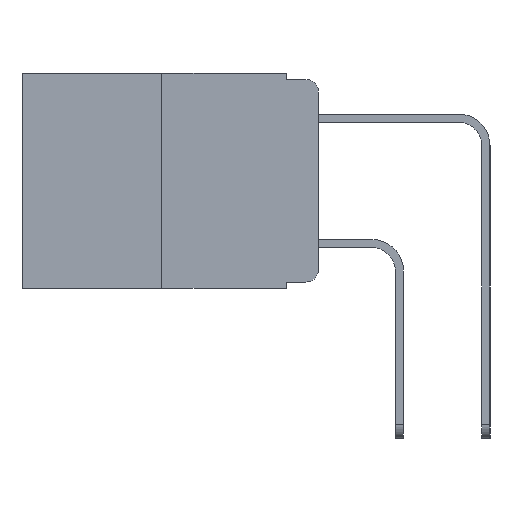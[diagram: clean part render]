
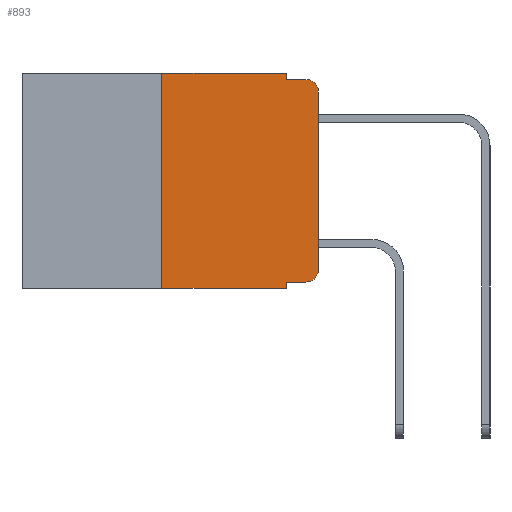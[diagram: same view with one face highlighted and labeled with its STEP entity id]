
A CAD part, left-side view. The second image highlights one B-rep face of the part: STEP entity #893.
In plain terms, the highlighted planar face has unit normal (-1, 0, 0).
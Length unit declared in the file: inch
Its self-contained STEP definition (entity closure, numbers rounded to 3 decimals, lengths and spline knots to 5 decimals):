
#57 = ORIENTED_EDGE ( 'NONE', *, *, #6435, .F. ) ;
#173 = CARTESIAN_POINT ( 'NONE',  ( 0., 0.051, -0.01 ) ) ;
#435 = DIRECTION ( 'NONE',  ( 0., 0., 1. ) ) ;
#617 = DIRECTION ( 'NONE',  ( 0., 0., -1. ) ) ;
#740 = DIRECTION ( 'NONE',  ( 0., -1., 0. ) ) ;
#786 = ORIENTED_EDGE ( 'NONE', *, *, #6871, .T. ) ;
#841 = ORIENTED_EDGE ( 'NONE', *, *, #5917, .T. ) ;
#893 = ADVANCED_FACE ( 'NONE', ( #14745 ), #947, .F. ) ;
#947 = PLANE ( 'NONE',  #5360 ) ;
#1218 = EDGE_CURVE ( 'NONE', #14982, #10370, #7694, .T. ) ;
#1317 = VECTOR ( 'NONE', #435, 39.37008 ) ;
#1763 = EDGE_LOOP ( 'NONE', ( #786, #841, #57, #3792, #8939, #8729, #2257, #1933, #3861, #8862 ) ) ;
#1921 = CIRCLE ( 'NONE', #11222, 0.02 ) ;
#1933 = ORIENTED_EDGE ( 'NONE', *, *, #4482, .F. ) ;
#2257 = ORIENTED_EDGE ( 'NONE', *, *, #1218, .T. ) ;
#2333 = DIRECTION ( 'NONE',  ( 0., 0., -1. ) ) ;
#2647 = CARTESIAN_POINT ( 'NONE',  ( 0., 0.02, -0.03 ) ) ;
#3167 = CARTESIAN_POINT ( 'NONE',  ( 0., 0., 0. ) ) ;
#3322 = CARTESIAN_POINT ( 'NONE',  ( 0., 0.02, -0.01 ) ) ;
#3792 = ORIENTED_EDGE ( 'NONE', *, *, #13071, .F. ) ;
#3861 = ORIENTED_EDGE ( 'NONE', *, *, #12521, .T. ) ;
#3961 = DIRECTION ( 'NONE',  ( 0., 0., -1. ) ) ;
#4212 = LINE ( 'NONE', #9651, #7552 ) ;
#4482 = EDGE_CURVE ( 'NONE', #14192, #10370, #9953, .T. ) ;
#4550 = CARTESIAN_POINT ( 'NONE',  ( 0., 0.02, -0.333 ) ) ;
#4889 = CIRCLE ( 'NONE', #15870, 0.02 ) ;
#4907 = DIRECTION ( 'NONE',  ( 1., 0., 0. ) ) ;
#4978 = VERTEX_POINT ( 'NONE', #3322 ) ;
#5306 = VERTEX_POINT ( 'NONE', #9014 ) ;
#5360 = AXIS2_PLACEMENT_3D ( 'NONE', #11099, #4907, #13503 ) ;
#5851 = DIRECTION ( 'NONE',  ( 0., -1., 0. ) ) ;
#5917 = EDGE_CURVE ( 'NONE', #10586, #4978, #1921, .T. ) ;
#6300 = CARTESIAN_POINT ( 'NONE',  ( 0., 0.051, 0. ) ) ;
#6374 = DIRECTION ( 'NONE',  ( -1., 0., 0. ) ) ;
#6435 = EDGE_CURVE ( 'NONE', #14594, #4978, #11565, .T. ) ;
#6600 = VECTOR ( 'NONE', #2333, 39.37008 ) ;
#6871 = EDGE_CURVE ( 'NONE', #10954, #10586, #8699, .T. ) ;
#7233 = LINE ( 'NONE', #9596, #10561 ) ;
#7552 = VECTOR ( 'NONE', #10809, 39.37008 ) ;
#7694 = LINE ( 'NONE', #8012, #13799 ) ;
#8012 = CARTESIAN_POINT ( 'NONE',  ( 0., 0.473, -0.343 ) ) ;
#8699 = LINE ( 'NONE', #3167, #11929 ) ;
#8729 = ORIENTED_EDGE ( 'NONE', *, *, #9023, .F. ) ;
#8862 = ORIENTED_EDGE ( 'NONE', *, *, #13226, .T. ) ;
#8863 = EDGE_CURVE ( 'NONE', #5306, #12124, #4212, .T. ) ;
#8939 = ORIENTED_EDGE ( 'NONE', *, *, #8863, .F. ) ;
#9014 = CARTESIAN_POINT ( 'NONE',  ( 0., 0.25, 0. ) ) ;
#9023 = EDGE_CURVE ( 'NONE', #14982, #5306, #14600, .T. ) ;
#9596 = CARTESIAN_POINT ( 'NONE',  ( 0., 0.051, 0. ) ) ;
#9635 = LINE ( 'NONE', #15685, #12432 ) ;
#9651 = CARTESIAN_POINT ( 'NONE',  ( 0., 0.473, 0. ) ) ;
#9659 = CARTESIAN_POINT ( 'NONE',  ( 0., 0.051, -0.343 ) ) ;
#9953 = LINE ( 'NONE', #11158, #6600 ) ;
#10370 = VERTEX_POINT ( 'NONE', #9659 ) ;
#10561 = VECTOR ( 'NONE', #617, 39.37008 ) ;
#10586 = VERTEX_POINT ( 'NONE', #11259 ) ;
#10794 = CARTESIAN_POINT ( 'NONE',  ( 0., 0., -0.313 ) ) ;
#10809 = DIRECTION ( 'NONE',  ( 0., -1., 0. ) ) ;
#10954 = VERTEX_POINT ( 'NONE', #10794 ) ;
#11099 = CARTESIAN_POINT ( 'NONE',  ( 0., 0.473, 0. ) ) ;
#11120 = CARTESIAN_POINT ( 'NONE',  ( 0., 0.25, -0.343 ) ) ;
#11158 = CARTESIAN_POINT ( 'NONE',  ( 0., 0.051, 0. ) ) ;
#11222 = AXIS2_PLACEMENT_3D ( 'NONE', #2647, #11419, #3961 ) ;
#11259 = CARTESIAN_POINT ( 'NONE',  ( 0., 0., -0.03 ) ) ;
#11419 = DIRECTION ( 'NONE',  ( -1., 0., 0. ) ) ;
#11565 = LINE ( 'NONE', #14419, #14384 ) ;
#11929 = VECTOR ( 'NONE', #13120, 39.37008 ) ;
#12124 = VERTEX_POINT ( 'NONE', #6300 ) ;
#12432 = VECTOR ( 'NONE', #740, 39.37008 ) ;
#12521 = EDGE_CURVE ( 'NONE', #14192, #14199, #9635, .T. ) ;
#12924 = DIRECTION ( 'NONE',  ( 0., -1., 0. ) ) ;
#13071 = EDGE_CURVE ( 'NONE', #12124, #14594, #7233, .T. ) ;
#13120 = DIRECTION ( 'NONE',  ( 0., 0., 1. ) ) ;
#13226 = EDGE_CURVE ( 'NONE', #14199, #10954, #4889, .T. ) ;
#13503 = DIRECTION ( 'NONE',  ( 0., 0., -1. ) ) ;
#13731 = CARTESIAN_POINT ( 'NONE',  ( 0., 0.02, -0.313 ) ) ;
#13799 = VECTOR ( 'NONE', #12924, 39.37008 ) ;
#14192 = VERTEX_POINT ( 'NONE', #14330 ) ;
#14199 = VERTEX_POINT ( 'NONE', #4550 ) ;
#14250 = CARTESIAN_POINT ( 'NONE',  ( 0., 0.25, 0. ) ) ;
#14330 = CARTESIAN_POINT ( 'NONE',  ( 0., 0.051, -0.333 ) ) ;
#14384 = VECTOR ( 'NONE', #5851, 39.37008 ) ;
#14419 = CARTESIAN_POINT ( 'NONE',  ( 0., 0.051, -0.01 ) ) ;
#14594 = VERTEX_POINT ( 'NONE', #173 ) ;
#14600 = LINE ( 'NONE', #14250, #1317 ) ;
#14745 = FACE_OUTER_BOUND ( 'NONE', #1763, .T. ) ;
#14933 = DIRECTION ( 'NONE',  ( 0., 0., -1. ) ) ;
#14982 = VERTEX_POINT ( 'NONE', #11120 ) ;
#15685 = CARTESIAN_POINT ( 'NONE',  ( 0., 0.051, -0.333 ) ) ;
#15870 = AXIS2_PLACEMENT_3D ( 'NONE', #13731, #6374, #14933 ) ;
